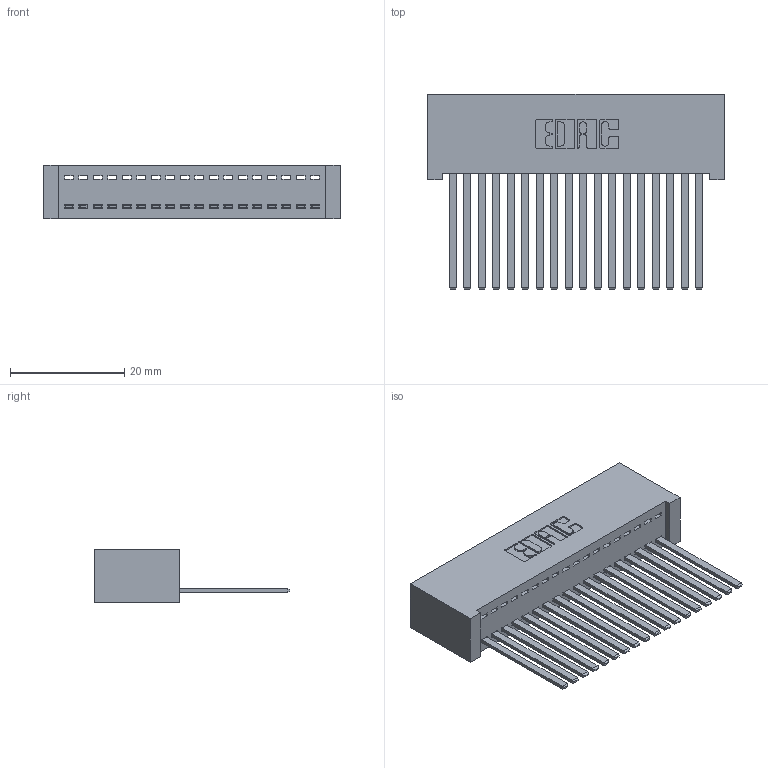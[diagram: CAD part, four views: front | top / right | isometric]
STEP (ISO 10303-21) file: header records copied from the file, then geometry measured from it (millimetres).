
FILE_DESCRIPTION (( 'STEP AP203' ), '1' );
FILE_NAME ('342-018-544-101.STEP', '2019-10-01T20:06:47', ( '' ), ( '' ), 'SwSTEP 2.0', 'SolidWorks 2016', '' );
FILE_SCHEMA (( 'CONFIG_CONTROL_DESIGN' ));
Length unit declared in the file: inch
Products named in the file (3): 342-018-544-101; 342 Part_Lugless; 345-292-001_345-293-144
Assembly tree (19 placements, depth 2):
  342-018-544-101
    342 Part_Lugless
    345-292-001_345-293-144  x18
Bounding box: 51.97 x 34.3 x 9.4 mm (x, y, z)
Volume: 5085.6 mm3; surface area: 7936.5 mm2
Topology: 19 solids, 19 shells, 1038 faces, 3119 edges, 2054 vertices
Faces by surface type: plane 746, cylinder 292
Entity records: 13515 total; most frequent: CARTESIAN_POINT 2340, ORIENTED_EDGE 2294, DIRECTION 2011, EDGE_CURVE 1147, VECTOR 1031, LINE 1031, VERTEX_POINT 762, AXIS2_PLACEMENT_3D 490
